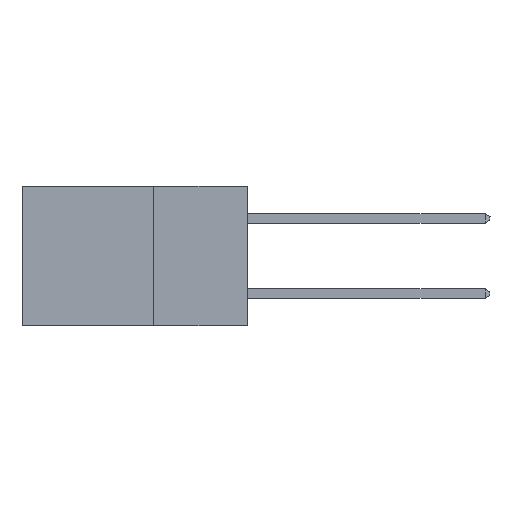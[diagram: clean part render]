
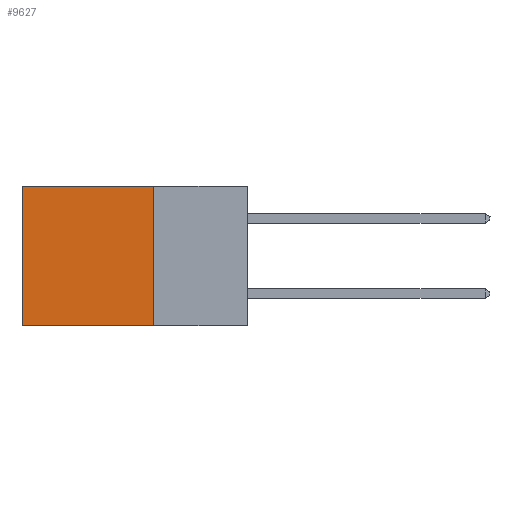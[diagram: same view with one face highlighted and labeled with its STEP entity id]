
A CAD part, left-side view. The second image highlights one B-rep face of the part: STEP entity #9627.
In plain terms, the highlighted planar face has unit normal (-1, 0, 0).
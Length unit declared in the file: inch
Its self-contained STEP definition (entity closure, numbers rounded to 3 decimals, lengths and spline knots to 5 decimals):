
#56 = VERTEX_POINT ( 'NONE', #8393 ) ;
#492 = VERTEX_POINT ( 'NONE', #8587 ) ;
#2616 = VECTOR ( 'NONE', #11330, 39.37008 ) ;
#2653 = CARTESIAN_POINT ( 'NONE',  ( 0.298, 0.25, 0. ) ) ;
#3247 = DIRECTION ( 'NONE',  ( 1., 0., 0. ) ) ;
#3282 = LINE ( 'NONE', #2653, #2616 ) ;
#5086 = DIRECTION ( 'NONE',  ( 0., 1., 0. ) ) ;
#7640 = EDGE_CURVE ( 'NONE', #492, #7998, #3282, .T. ) ;
#7998 = VERTEX_POINT ( 'NONE', #19364 ) ;
#8227 = FACE_OUTER_BOUND ( 'NONE', #22621, .T. ) ;
#8393 = CARTESIAN_POINT ( 'NONE',  ( 0.298, 0.6, 0. ) ) ;
#8587 = CARTESIAN_POINT ( 'NONE',  ( 0.298, 0.25, 0. ) ) ;
#8688 = CARTESIAN_POINT ( 'NONE',  ( 0.298, 0.25, 0. ) ) ;
#8890 = ORIENTED_EDGE ( 'NONE', *, *, #7640, .F. ) ;
#9627 = ADVANCED_FACE ( 'NONE', ( #8227 ), #9855, .F. ) ;
#9855 = PLANE ( 'NONE',  #10975 ) ;
#10975 = AXIS2_PLACEMENT_3D ( 'NONE', #16250, #3247, #27310 ) ;
#11298 = ORIENTED_EDGE ( 'NONE', *, *, #27741, .F. ) ;
#11330 = DIRECTION ( 'NONE',  ( 0., 0., -1. ) ) ;
#11610 = LINE ( 'NONE', #18700, #13959 ) ;
#12267 = LINE ( 'NONE', #19526, #21349 ) ;
#13959 = VECTOR ( 'NONE', #25103, 39.37008 ) ;
#16250 = CARTESIAN_POINT ( 'NONE',  ( 0.298, 0.25, 0. ) ) ;
#16432 = EDGE_CURVE ( 'NONE', #492, #56, #25852, .T. ) ;
#18700 = CARTESIAN_POINT ( 'NONE',  ( 0.298, 0.6, 0. ) ) ;
#19364 = CARTESIAN_POINT ( 'NONE',  ( 0.298, 0.25, -0.37 ) ) ;
#19526 = CARTESIAN_POINT ( 'NONE',  ( 0.298, 0.25, -0.37 ) ) ;
#20090 = VECTOR ( 'NONE', #5086, 39.37008 ) ;
#20104 = ORIENTED_EDGE ( 'NONE', *, *, #27202, .T. ) ;
#21349 = VECTOR ( 'NONE', #21420, 39.37008 ) ;
#21420 = DIRECTION ( 'NONE',  ( 0., 1., 0. ) ) ;
#22621 = EDGE_LOOP ( 'NONE', ( #20104, #11298, #8890, #25633 ) ) ;
#25103 = DIRECTION ( 'NONE',  ( 0., 0., -1. ) ) ;
#25633 = ORIENTED_EDGE ( 'NONE', *, *, #16432, .T. ) ;
#25852 = LINE ( 'NONE', #8688, #20090 ) ;
#26117 = VERTEX_POINT ( 'NONE', #26786 ) ;
#26786 = CARTESIAN_POINT ( 'NONE',  ( 0.298, 0.6, -0.37 ) ) ;
#27202 = EDGE_CURVE ( 'NONE', #56, #26117, #11610, .T. ) ;
#27310 = DIRECTION ( 'NONE',  ( 0., 0., -1. ) ) ;
#27741 = EDGE_CURVE ( 'NONE', #7998, #26117, #12267, .T. ) ;
